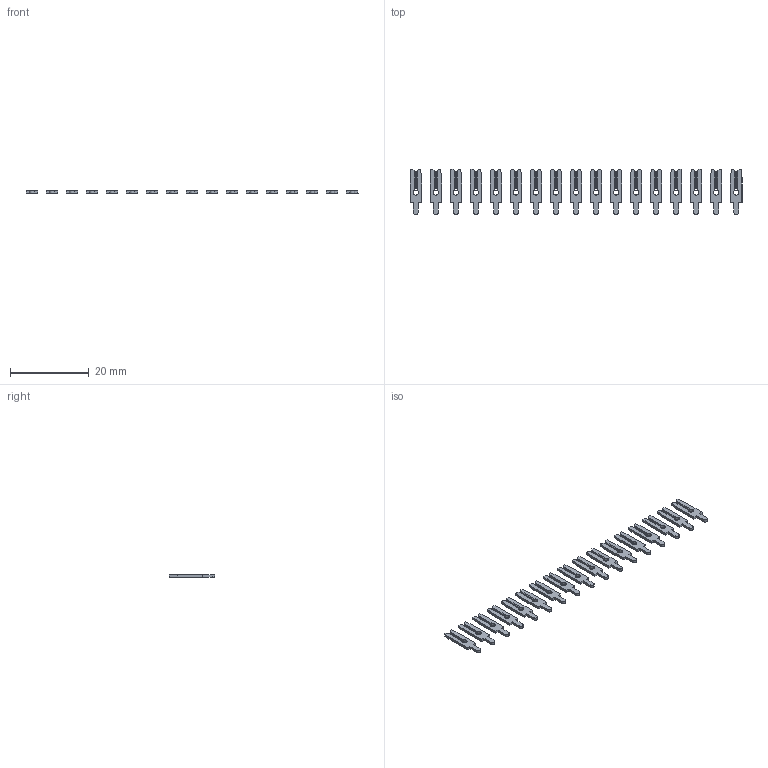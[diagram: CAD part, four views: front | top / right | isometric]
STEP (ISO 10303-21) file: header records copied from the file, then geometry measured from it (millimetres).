
FILE_DESCRIPTION (( 'STEP AP203' ), '1' );
FILE_NAME ('103-017-250-200.STEP', '2020-04-09T20:25:55', ( '' ), ( '' ), 'SwSTEP 2.0', 'SolidWorks 2016', '' );
FILE_SCHEMA (( 'CONFIG_CONTROL_DESIGN' ));
Length unit declared in the file: inch
Products named in the file (2): 103-017-250-200; 100-290-001_100-290-250
Assembly tree (17 placements, depth 2):
  103-017-250-200
    100-290-001_100-290-250  x17
Bounding box: 84.2 x 11.48 x 0.66 mm (x, y, z)
Volume: 265.3 mm3; surface area: 1246.9 mm2
Topology: 17 solids, 17 shells, 408 faces, 1122 edges, 748 vertices
Faces by surface type: plane 340, cylinder 68
Entity records: 1470 total; most frequent: CARTESIAN_POINT 166, DIRECTION 158, ORIENTED_EDGE 132, EDGE_CURVE 66, LINE 54, VECTOR 54, AXIS2_PLACEMENT_3D 52, LOCAL_TIME 44
